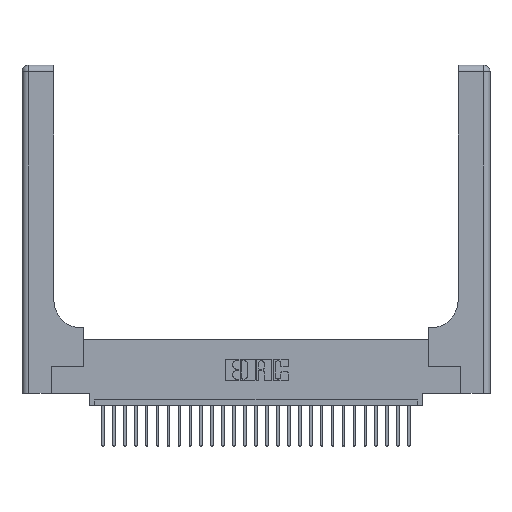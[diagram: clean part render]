
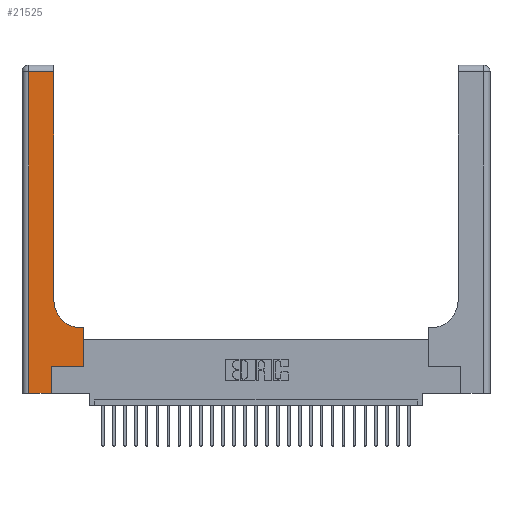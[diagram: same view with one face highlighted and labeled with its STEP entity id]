
A CAD part, top view. The second image highlights one B-rep face of the part: STEP entity #21525.
In plain terms, the highlighted planar face has unit normal (0, 0, 1).
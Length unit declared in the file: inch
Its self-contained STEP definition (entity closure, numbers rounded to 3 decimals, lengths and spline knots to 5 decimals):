
#121 = DIRECTION ( 'NONE',  ( 0., 1., 0. ) ) ;
#229 = ORIENTED_EDGE ( 'NONE', *, *, #1214, .T. ) ;
#836 = LINE ( 'NONE', #15615, #10926 ) ;
#1180 = AXIS2_PLACEMENT_3D ( 'NONE', #6255, #21935, #12996 ) ;
#1214 = EDGE_CURVE ( 'NONE', #5156, #2164, #5681, .T. ) ;
#1466 = CARTESIAN_POINT ( 'NONE',  ( 0.2915, 0.6, 0.37 ) ) ;
#1689 = PLANE ( 'NONE',  #1180 ) ;
#1699 = LINE ( 'NONE', #1466, #27192 ) ;
#2164 = VERTEX_POINT ( 'NONE', #13638 ) ;
#2239 = DIRECTION ( 'NONE',  ( 1., 0., 0. ) ) ;
#2628 = ORIENTED_EDGE ( 'NONE', *, *, #17645, .T. ) ;
#2648 = CARTESIAN_POINT ( 'NONE',  ( 0.06, 2.94, 0.37 ) ) ;
#3339 = ORIENTED_EDGE ( 'NONE', *, *, #16179, .T. ) ;
#4033 = CARTESIAN_POINT ( 'NONE',  ( 0.5585, 0.25, 0.37 ) ) ;
#4293 = EDGE_CURVE ( 'NONE', #23389, #14329, #11087, .T. ) ;
#4560 = DIRECTION ( 'NONE',  ( 0., 0., -1. ) ) ;
#5145 = VECTOR ( 'NONE', #8583, 39.37008 ) ;
#5156 = VERTEX_POINT ( 'NONE', #14265 ) ;
#5681 = CIRCLE ( 'NONE', #19216, 0.25 ) ;
#6094 = DIRECTION ( 'NONE',  ( 1., 0., 0. ) ) ;
#6255 = CARTESIAN_POINT ( 'NONE',  ( 0., 3., 0.37 ) ) ;
#6664 = LINE ( 'NONE', #19556, #17922 ) ;
#7083 = VECTOR ( 'NONE', #19696, 39.37008 ) ;
#7398 = VERTEX_POINT ( 'NONE', #11029 ) ;
#7715 = ORIENTED_EDGE ( 'NONE', *, *, #25344, .T. ) ;
#8530 = CARTESIAN_POINT ( 'NONE',  ( 0., 2.94, 0.37 ) ) ;
#8583 = DIRECTION ( 'NONE',  ( 0., 1., 0. ) ) ;
#9446 = VERTEX_POINT ( 'NONE', #26675 ) ;
#9481 = CARTESIAN_POINT ( 'NONE',  ( 0.5585, 0.25, 0.37 ) ) ;
#10050 = CARTESIAN_POINT ( 'NONE',  ( 0.269, 0.25, 0.37 ) ) ;
#10087 = DIRECTION ( 'NONE',  ( -1., 0., 0. ) ) ;
#10389 = VERTEX_POINT ( 'NONE', #2648 ) ;
#10603 = VECTOR ( 'NONE', #121, 39.37008 ) ;
#10621 = ORIENTED_EDGE ( 'NONE', *, *, #21566, .T. ) ;
#10926 = VECTOR ( 'NONE', #2239, 39.37008 ) ;
#11029 = CARTESIAN_POINT ( 'NONE',  ( 0.2915, 2.94, 0.37 ) ) ;
#11087 = LINE ( 'NONE', #4033, #5145 ) ;
#11157 = CARTESIAN_POINT ( 'NONE',  ( 0.2915, 3., 0.37 ) ) ;
#11557 = EDGE_LOOP ( 'NONE', ( #27287, #15262, #2628, #7715, #3339, #10621, #26410, #16265, #229 ) ) ;
#11690 = CARTESIAN_POINT ( 'NONE',  ( 0.269, 0., 0.37 ) ) ;
#12781 = VERTEX_POINT ( 'NONE', #10050 ) ;
#12996 = DIRECTION ( 'NONE',  ( -1., 0., 0. ) ) ;
#13124 = EDGE_CURVE ( 'NONE', #7398, #10389, #18195, .T. ) ;
#13638 = CARTESIAN_POINT ( 'NONE',  ( 0.2915, 0.85, 0.37 ) ) ;
#13650 = EDGE_CURVE ( 'NONE', #14329, #5156, #1699, .T. ) ;
#14265 = CARTESIAN_POINT ( 'NONE',  ( 0.5415, 0.6, 0.37 ) ) ;
#14329 = VERTEX_POINT ( 'NONE', #26393 ) ;
#15262 = ORIENTED_EDGE ( 'NONE', *, *, #13124, .T. ) ;
#15336 = DIRECTION ( 'NONE',  ( -1., 0., 0. ) ) ;
#15615 = CARTESIAN_POINT ( 'NONE',  ( 0.269, 0.25, 0.37 ) ) ;
#15836 = FACE_OUTER_BOUND ( 'NONE', #11557, .T. ) ;
#16179 = EDGE_CURVE ( 'NONE', #17362, #12781, #18716, .T. ) ;
#16265 = ORIENTED_EDGE ( 'NONE', *, *, #13650, .T. ) ;
#17362 = VERTEX_POINT ( 'NONE', #23141 ) ;
#17645 = EDGE_CURVE ( 'NONE', #10389, #9446, #25261, .T. ) ;
#17922 = VECTOR ( 'NONE', #6094, 39.37008 ) ;
#18044 = CARTESIAN_POINT ( 'NONE',  ( 0.5415, 0.85, 0.37 ) ) ;
#18194 = DIRECTION ( 'NONE',  ( 0., -1., 0. ) ) ;
#18195 = LINE ( 'NONE', #8530, #27947 ) ;
#18716 = LINE ( 'NONE', #11690, #7083 ) ;
#19216 = AXIS2_PLACEMENT_3D ( 'NONE', #18044, #4560, #20563 ) ;
#19556 = CARTESIAN_POINT ( 'NONE',  ( 0., 0., 0.37 ) ) ;
#19696 = DIRECTION ( 'NONE',  ( 0., 1., 0. ) ) ;
#20563 = DIRECTION ( 'NONE',  ( 1., 0., 0. ) ) ;
#21525 = ADVANCED_FACE ( 'NONE', ( #15836 ), #1689, .F. ) ;
#21566 = EDGE_CURVE ( 'NONE', #12781, #23389, #836, .T. ) ;
#21935 = DIRECTION ( 'NONE',  ( 0., 0., -1. ) ) ;
#22444 = EDGE_CURVE ( 'NONE', #2164, #7398, #28868, .T. ) ;
#23141 = CARTESIAN_POINT ( 'NONE',  ( 0.269, 0., 0.37 ) ) ;
#23389 = VERTEX_POINT ( 'NONE', #9481 ) ;
#23556 = VECTOR ( 'NONE', #18194, 39.37008 ) ;
#25261 = LINE ( 'NONE', #26963, #23556 ) ;
#25344 = EDGE_CURVE ( 'NONE', #9446, #17362, #6664, .T. ) ;
#26393 = CARTESIAN_POINT ( 'NONE',  ( 0.5585, 0.6, 0.37 ) ) ;
#26410 = ORIENTED_EDGE ( 'NONE', *, *, #4293, .T. ) ;
#26675 = CARTESIAN_POINT ( 'NONE',  ( 0.06, 0., 0.37 ) ) ;
#26963 = CARTESIAN_POINT ( 'NONE',  ( 0.06, 3., 0.37 ) ) ;
#27192 = VECTOR ( 'NONE', #10087, 39.37008 ) ;
#27287 = ORIENTED_EDGE ( 'NONE', *, *, #22444, .T. ) ;
#27947 = VECTOR ( 'NONE', #15336, 39.37008 ) ;
#28868 = LINE ( 'NONE', #11157, #10603 ) ;
